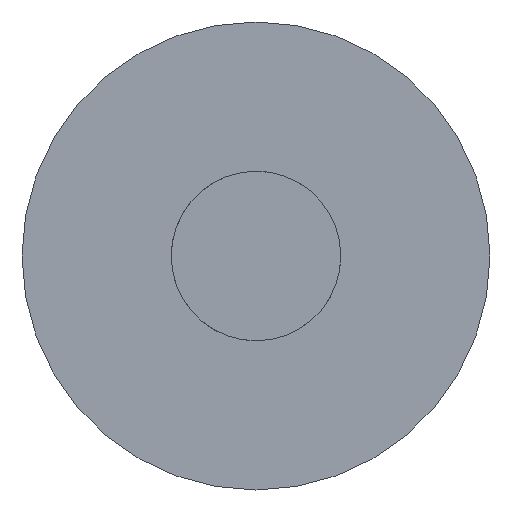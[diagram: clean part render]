
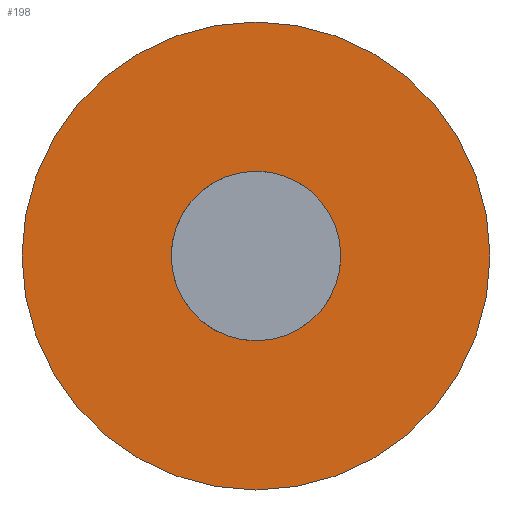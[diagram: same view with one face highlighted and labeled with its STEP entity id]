
A CAD part, left-side view. The second image highlights one B-rep face of the part: STEP entity #198.
In plain terms, the highlighted planar face has unit normal (-1, 0, 0).
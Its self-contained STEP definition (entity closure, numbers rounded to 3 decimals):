
#12 = CARTESIAN_POINT ( 'NONE',  ( -5., 0., 0. ) ) ;
#17 = PLANE ( 'NONE',  #238 ) ;
#33 = CARTESIAN_POINT ( 'NONE',  ( -5., 0., 8. ) ) ;
#44 = FACE_OUTER_BOUND ( 'NONE', #258, .T. ) ;
#50 = AXIS2_PLACEMENT_3D ( 'NONE', #12, #102, #136 ) ;
#84 = CARTESIAN_POINT ( 'NONE',  ( -5., 0., 0. ) ) ;
#86 = CARTESIAN_POINT ( 'NONE',  ( -5., 0., 0. ) ) ;
#99 = EDGE_CURVE ( 'NONE', #220, #220, #226, .T. ) ;
#102 = DIRECTION ( 'NONE',  ( -1., 0., 0. ) ) ;
#136 = DIRECTION ( 'NONE',  ( 0., 0., 1. ) ) ;
#155 = FACE_BOUND ( 'NONE', #216, .T. ) ;
#161 = AXIS2_PLACEMENT_3D ( 'NONE', #86, #234, #187 ) ;
#167 = ORIENTED_EDGE ( 'NONE', *, *, #99, .T. ) ;
#168 = EDGE_CURVE ( 'NONE', #213, #213, #274, .T. ) ;
#187 = DIRECTION ( 'NONE',  ( 0., 0., 1. ) ) ;
#188 = DIRECTION ( 'NONE',  ( 0., 0., 1. ) ) ;
#198 = ADVANCED_FACE ( 'NONE', ( #155, #44 ), #17, .T. ) ;
#199 = ORIENTED_EDGE ( 'NONE', *, *, #168, .F. ) ;
#212 = CARTESIAN_POINT ( 'NONE',  ( -5., 0., 2.9 ) ) ;
#213 = VERTEX_POINT ( 'NONE', #212 ) ;
#216 = EDGE_LOOP ( 'NONE', ( #199 ) ) ;
#220 = VERTEX_POINT ( 'NONE', #33 ) ;
#226 = CIRCLE ( 'NONE', #50, 8. ) ;
#234 = DIRECTION ( 'NONE',  ( -1., 0., 0. ) ) ;
#238 = AXIS2_PLACEMENT_3D ( 'NONE', #84, #256, #188 ) ;
#256 = DIRECTION ( 'NONE',  ( -1., 0., 0. ) ) ;
#258 = EDGE_LOOP ( 'NONE', ( #167 ) ) ;
#274 = CIRCLE ( 'NONE', #161, 2.9 ) ;
